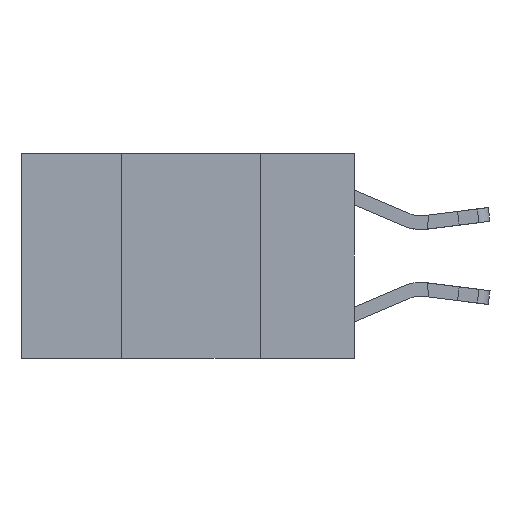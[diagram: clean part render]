
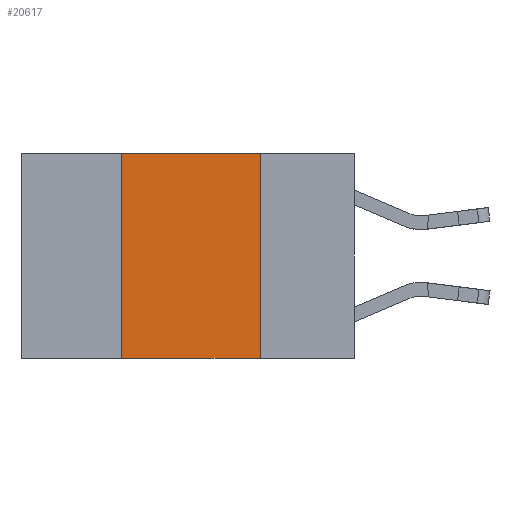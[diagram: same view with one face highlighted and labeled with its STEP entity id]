
A CAD part, left-side view. The second image highlights one B-rep face of the part: STEP entity #20617.
In plain terms, the highlighted planar face has unit normal (-1, 0, 0).
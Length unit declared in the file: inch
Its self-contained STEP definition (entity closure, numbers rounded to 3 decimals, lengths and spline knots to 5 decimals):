
#547 = EDGE_CURVE ( 'NONE', #10549, #16081, #9367, .T. ) ;
#1779 = CARTESIAN_POINT ( 'NONE',  ( 0., 0.17, -0.37 ) ) ;
#2740 = VERTEX_POINT ( 'NONE', #14009 ) ;
#3275 = ORIENTED_EDGE ( 'NONE', *, *, #12074, .F. ) ;
#3561 = ORIENTED_EDGE ( 'NONE', *, *, #20382, .T. ) ;
#5774 = DIRECTION ( 'NONE',  ( 0., 0., 1. ) ) ;
#6993 = DIRECTION ( 'NONE',  ( 1., 0., 0. ) ) ;
#6997 = CARTESIAN_POINT ( 'NONE',  ( 0., 0.17, 0. ) ) ;
#8818 = DIRECTION ( 'NONE',  ( 0., 0., -1. ) ) ;
#9172 = ORIENTED_EDGE ( 'NONE', *, *, #547, .F. ) ;
#9198 = LINE ( 'NONE', #22559, #18839 ) ;
#9236 = CARTESIAN_POINT ( 'NONE',  ( 0., 0.42, -0.37 ) ) ;
#9367 = LINE ( 'NONE', #6997, #9934 ) ;
#9934 = VECTOR ( 'NONE', #8818, 39.37008 ) ;
#9977 = VERTEX_POINT ( 'NONE', #9236 ) ;
#10549 = VERTEX_POINT ( 'NONE', #17922 ) ;
#10686 = CARTESIAN_POINT ( 'NONE',  ( 0., 0.6, 0. ) ) ;
#11364 = LINE ( 'NONE', #18455, #16187 ) ;
#11714 = DIRECTION ( 'NONE',  ( 0., -1., 0. ) ) ;
#12074 = EDGE_CURVE ( 'NONE', #2740, #10549, #13588, .T. ) ;
#13588 = LINE ( 'NONE', #10686, #14175 ) ;
#14009 = CARTESIAN_POINT ( 'NONE',  ( 0., 0.42, 0. ) ) ;
#14175 = VECTOR ( 'NONE', #23320, 39.37008 ) ;
#16081 = VERTEX_POINT ( 'NONE', #1779 ) ;
#16187 = VECTOR ( 'NONE', #5774, 39.37008 ) ;
#17830 = CARTESIAN_POINT ( 'NONE',  ( 0., 0.6, 0. ) ) ;
#17922 = CARTESIAN_POINT ( 'NONE',  ( 0., 0.17, 0. ) ) ;
#18455 = CARTESIAN_POINT ( 'NONE',  ( 0., 0.42, 0. ) ) ;
#18543 = FACE_OUTER_BOUND ( 'NONE', #22530, .T. ) ;
#18839 = VECTOR ( 'NONE', #11714, 39.37008 ) ;
#19650 = DIRECTION ( 'NONE',  ( 0., 0., -1. ) ) ;
#20382 = EDGE_CURVE ( 'NONE', #9977, #16081, #9198, .T. ) ;
#20617 = ADVANCED_FACE ( 'NONE', ( #18543 ), #23188, .F. ) ;
#21023 = AXIS2_PLACEMENT_3D ( 'NONE', #17830, #6993, #19650 ) ;
#21523 = ORIENTED_EDGE ( 'NONE', *, *, #22824, .F. ) ;
#22530 = EDGE_LOOP ( 'NONE', ( #9172, #3275, #21523, #3561 ) ) ;
#22559 = CARTESIAN_POINT ( 'NONE',  ( 0., 0.6, -0.37 ) ) ;
#22824 = EDGE_CURVE ( 'NONE', #9977, #2740, #11364, .T. ) ;
#23188 = PLANE ( 'NONE',  #21023 ) ;
#23320 = DIRECTION ( 'NONE',  ( 0., -1., 0. ) ) ;
